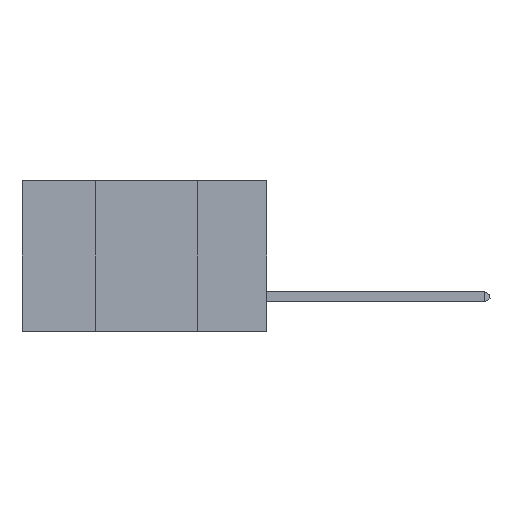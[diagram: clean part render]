
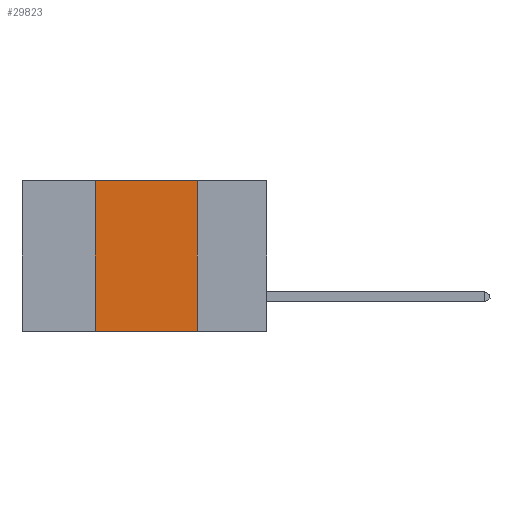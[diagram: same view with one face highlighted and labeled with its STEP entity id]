
A CAD part, left-side view. The second image highlights one B-rep face of the part: STEP entity #29823.
In plain terms, the highlighted planar face has unit normal (-1, 0, 0).
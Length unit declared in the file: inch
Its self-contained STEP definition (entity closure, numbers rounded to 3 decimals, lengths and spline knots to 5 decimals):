
#96 = LINE ( 'NONE', #19546, #14189 ) ;
#1277 = VECTOR ( 'NONE', #35773, 39.37008 ) ;
#1879 = DIRECTION ( 'NONE',  ( 0., 0., 1. ) ) ;
#2555 = VECTOR ( 'NONE', #1879, 39.37008 ) ;
#3663 = PLANE ( 'NONE',  #35142 ) ;
#3945 = CARTESIAN_POINT ( 'NONE',  ( 0., 0.6, 0. ) ) ;
#4316 = LINE ( 'NONE', #12986, #1277 ) ;
#5015 = CARTESIAN_POINT ( 'NONE',  ( 0., 0.17, 0. ) ) ;
#6121 = VECTOR ( 'NONE', #23359, 39.37008 ) ;
#6347 = ORIENTED_EDGE ( 'NONE', *, *, #10988, .F. ) ;
#6421 = ORIENTED_EDGE ( 'NONE', *, *, #33401, .T. ) ;
#6554 = EDGE_CURVE ( 'NONE', #19304, #33484, #24214, .T. ) ;
#8074 = CARTESIAN_POINT ( 'NONE',  ( 0., 0.42, 0. ) ) ;
#10988 = EDGE_CURVE ( 'NONE', #33484, #32104, #96, .T. ) ;
#12986 = CARTESIAN_POINT ( 'NONE',  ( 0., 0.6, -0.37 ) ) ;
#13244 = FACE_OUTER_BOUND ( 'NONE', #37582, .T. ) ;
#14189 = VECTOR ( 'NONE', #31809, 39.37008 ) ;
#15803 = ORIENTED_EDGE ( 'NONE', *, *, #6554, .F. ) ;
#19304 = VERTEX_POINT ( 'NONE', #31609 ) ;
#19546 = CARTESIAN_POINT ( 'NONE',  ( 0., 0.17, 0. ) ) ;
#20276 = CARTESIAN_POINT ( 'NONE',  ( 0., 0.6, 0. ) ) ;
#23359 = DIRECTION ( 'NONE',  ( 0., -1., 0. ) ) ;
#23528 = ORIENTED_EDGE ( 'NONE', *, *, #31189, .F. ) ;
#24214 = LINE ( 'NONE', #3945, #6121 ) ;
#25700 = CARTESIAN_POINT ( 'NONE',  ( 0., 0.17, -0.37 ) ) ;
#29762 = DIRECTION ( 'NONE',  ( 0., 0., -1. ) ) ;
#29823 = ADVANCED_FACE ( 'NONE', ( #13244 ), #3663, .F. ) ;
#31189 = EDGE_CURVE ( 'NONE', #31423, #19304, #36670, .T. ) ;
#31423 = VERTEX_POINT ( 'NONE', #38101 ) ;
#31609 = CARTESIAN_POINT ( 'NONE',  ( 0., 0.42, 0. ) ) ;
#31809 = DIRECTION ( 'NONE',  ( 0., 0., -1. ) ) ;
#32104 = VERTEX_POINT ( 'NONE', #25700 ) ;
#33401 = EDGE_CURVE ( 'NONE', #31423, #32104, #4316, .T. ) ;
#33484 = VERTEX_POINT ( 'NONE', #5015 ) ;
#35142 = AXIS2_PLACEMENT_3D ( 'NONE', #20276, #39587, #29762 ) ;
#35773 = DIRECTION ( 'NONE',  ( 0., -1., 0. ) ) ;
#36670 = LINE ( 'NONE', #8074, #2555 ) ;
#37582 = EDGE_LOOP ( 'NONE', ( #6347, #15803, #23528, #6421 ) ) ;
#38101 = CARTESIAN_POINT ( 'NONE',  ( 0., 0.42, -0.37 ) ) ;
#39587 = DIRECTION ( 'NONE',  ( 1., 0., 0. ) ) ;
